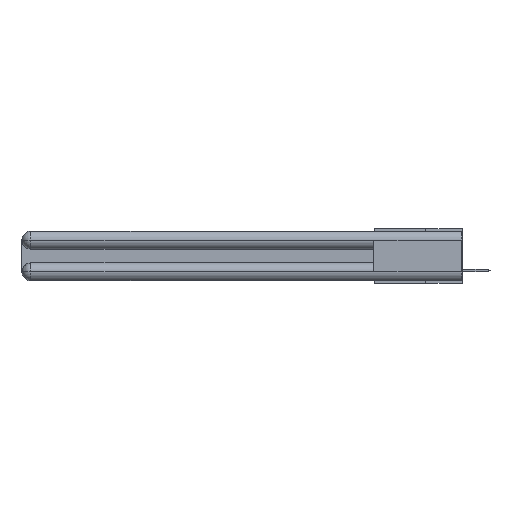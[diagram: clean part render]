
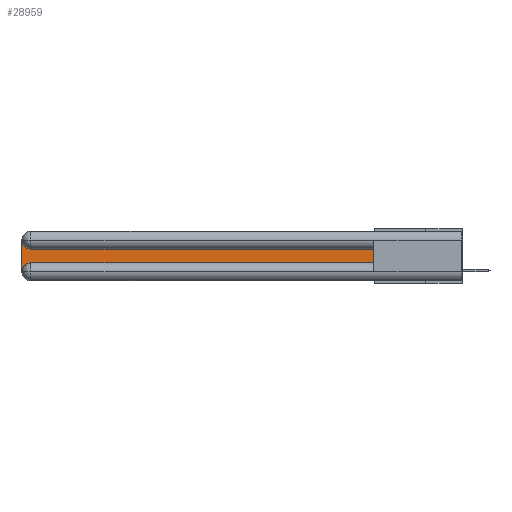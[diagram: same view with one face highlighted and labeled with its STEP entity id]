
A CAD part, left-side view. The second image highlights one B-rep face of the part: STEP entity #28959.
In plain terms, the highlighted planar face has unit normal (-1, 0, 0).
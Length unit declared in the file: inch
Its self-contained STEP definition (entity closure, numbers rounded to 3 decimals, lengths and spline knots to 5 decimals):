
#448 = AXIS2_PLACEMENT_3D ( 'NONE', #7747, #22085, #26380 ) ;
#683 = VERTEX_POINT ( 'NONE', #17441 ) ;
#1097 = DIRECTION ( 'NONE',  ( 0., 0., -1. ) ) ;
#1181 = CARTESIAN_POINT ( 'NONE',  ( 0.075, 3., -0.2775 ) ) ;
#1657 = VECTOR ( 'NONE', #23651, 39.37008 ) ;
#4012 = CARTESIAN_POINT ( 'NONE',  ( 0.075, 2.94, -0.2775 ) ) ;
#4064 = EDGE_CURVE ( 'NONE', #5401, #683, #16824, .T. ) ;
#4286 = VERTEX_POINT ( 'NONE', #18510 ) ;
#4314 = VECTOR ( 'NONE', #22620, 39.37008 ) ;
#4368 = ORIENTED_EDGE ( 'NONE', *, *, #8021, .T. ) ;
#5401 = VERTEX_POINT ( 'NONE', #26686 ) ;
#5415 = EDGE_LOOP ( 'NONE', ( #11652, #28098, #6578, #10138, #14211, #4368 ) ) ;
#6420 = LINE ( 'NONE', #8363, #25750 ) ;
#6578 = ORIENTED_EDGE ( 'NONE', *, *, #20686, .T. ) ;
#7351 = CARTESIAN_POINT ( 'NONE',  ( 0.075, 0.6, -0.2175 ) ) ;
#7747 = CARTESIAN_POINT ( 'NONE',  ( 0.075, 2.94, -0.0625 ) ) ;
#8021 = EDGE_CURVE ( 'NONE', #28109, #4286, #11850, .T. ) ;
#8363 = CARTESIAN_POINT ( 'NONE',  ( 0.075, 3., -0.2175 ) ) ;
#9390 = CIRCLE ( 'NONE', #28467, 0.06 ) ;
#10138 = ORIENTED_EDGE ( 'NONE', *, *, #24897, .T. ) ;
#10698 = VECTOR ( 'NONE', #29784, 39.37008 ) ;
#11175 = CARTESIAN_POINT ( 'NONE',  ( 0.075, 0.6, -0.2175 ) ) ;
#11652 = ORIENTED_EDGE ( 'NONE', *, *, #17122, .T. ) ;
#11850 = LINE ( 'NONE', #7351, #1657 ) ;
#11861 = VERTEX_POINT ( 'NONE', #26016 ) ;
#13907 = VERTEX_POINT ( 'NONE', #1181 ) ;
#14211 = ORIENTED_EDGE ( 'NONE', *, *, #26532, .T. ) ;
#15346 = CARTESIAN_POINT ( 'NONE',  ( 0.075, 0.6, -0.1225 ) ) ;
#15468 = DIRECTION ( 'NONE',  ( 0., 0., -1. ) ) ;
#15610 = DIRECTION ( 'NONE',  ( 0., 0., -1. ) ) ;
#15809 = CARTESIAN_POINT ( 'NONE',  ( 0.075, 3., -0.1225 ) ) ;
#16027 = CARTESIAN_POINT ( 'NONE',  ( 0.075, 0.6, -0.2175 ) ) ;
#16824 = CIRCLE ( 'NONE', #448, 0.06 ) ;
#17122 = EDGE_CURVE ( 'NONE', #4286, #5401, #24677, .T. ) ;
#17441 = CARTESIAN_POINT ( 'NONE',  ( 0.075, 3., -0.0625 ) ) ;
#18378 = PLANE ( 'NONE',  #26165 ) ;
#18510 = CARTESIAN_POINT ( 'NONE',  ( 0.075, 0.6, -0.1225 ) ) ;
#20686 = EDGE_CURVE ( 'NONE', #683, #13907, #6420, .T. ) ;
#22085 = DIRECTION ( 'NONE',  ( 1., 0., 0. ) ) ;
#22620 = DIRECTION ( 'NONE',  ( 0., 1., 0. ) ) ;
#23560 = FACE_OUTER_BOUND ( 'NONE', #5415, .T. ) ;
#23651 = DIRECTION ( 'NONE',  ( 0., 0., 1. ) ) ;
#24669 = DIRECTION ( 'NONE',  ( 1., 0., 0. ) ) ;
#24677 = LINE ( 'NONE', #15346, #4314 ) ;
#24897 = EDGE_CURVE ( 'NONE', #13907, #11861, #9390, .T. ) ;
#25750 = VECTOR ( 'NONE', #1097, 39.37008 ) ;
#26016 = CARTESIAN_POINT ( 'NONE',  ( 0.075, 2.94, -0.2175 ) ) ;
#26165 = AXIS2_PLACEMENT_3D ( 'NONE', #15809, #29644, #15610 ) ;
#26380 = DIRECTION ( 'NONE',  ( 0., 0., -1. ) ) ;
#26532 = EDGE_CURVE ( 'NONE', #11861, #28109, #28983, .T. ) ;
#26686 = CARTESIAN_POINT ( 'NONE',  ( 0.075, 2.94, -0.1225 ) ) ;
#28098 = ORIENTED_EDGE ( 'NONE', *, *, #4064, .T. ) ;
#28109 = VERTEX_POINT ( 'NONE', #16027 ) ;
#28467 = AXIS2_PLACEMENT_3D ( 'NONE', #4012, #24669, #15468 ) ;
#28959 = ADVANCED_FACE ( 'NONE', ( #23560 ), #18378, .F. ) ;
#28983 = LINE ( 'NONE', #11175, #10698 ) ;
#29644 = DIRECTION ( 'NONE',  ( 1., 0., 0. ) ) ;
#29784 = DIRECTION ( 'NONE',  ( 0., -1., 0. ) ) ;
